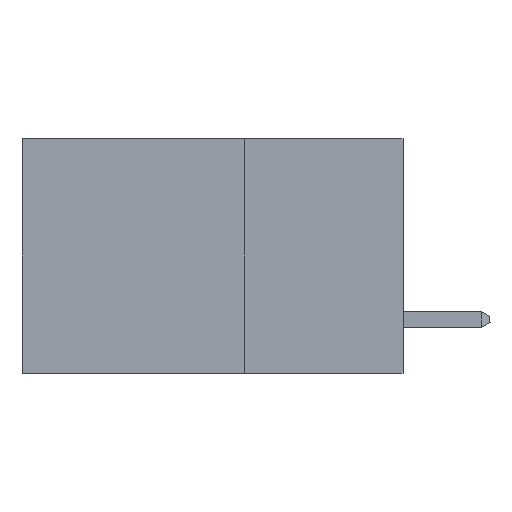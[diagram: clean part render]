
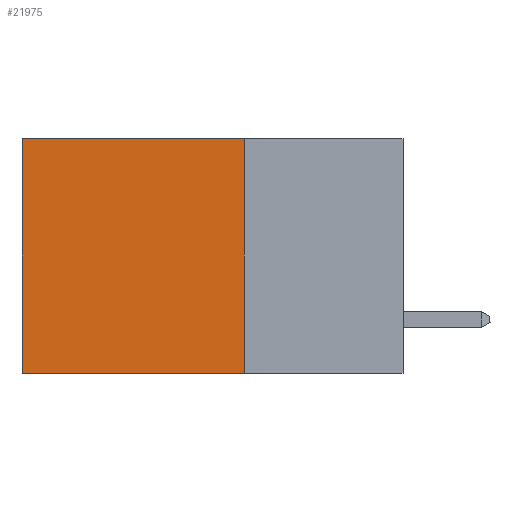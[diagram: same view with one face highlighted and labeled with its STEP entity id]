
A CAD part, left-side view. The second image highlights one B-rep face of the part: STEP entity #21975.
In plain terms, the highlighted planar face has unit normal (-1, 0, 0).
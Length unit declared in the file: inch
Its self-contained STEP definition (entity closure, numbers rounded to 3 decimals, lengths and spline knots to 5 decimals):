
#551 = EDGE_CURVE ( 'NONE', #24679, #6887, #25956, .T. ) ;
#995 = CARTESIAN_POINT ( 'NONE',  ( 0.2875, 0.25, -0.37 ) ) ;
#1259 = DIRECTION ( 'NONE',  ( 1., 0., 0. ) ) ;
#3183 = VECTOR ( 'NONE', #36712, 39.37008 ) ;
#5086 = DIRECTION ( 'NONE',  ( 0., 0., -1. ) ) ;
#6780 = VECTOR ( 'NONE', #36446, 39.37008 ) ;
#6887 = VERTEX_POINT ( 'NONE', #22088 ) ;
#7723 = DIRECTION ( 'NONE',  ( 0., 1., 0. ) ) ;
#8922 = VERTEX_POINT ( 'NONE', #23447 ) ;
#12280 = EDGE_CURVE ( 'NONE', #24679, #21773, #35137, .T. ) ;
#16312 = CARTESIAN_POINT ( 'NONE',  ( 0.2875, 0.6, 0. ) ) ;
#17929 = VECTOR ( 'NONE', #7723, 39.37008 ) ;
#19076 = EDGE_CURVE ( 'NONE', #6887, #8922, #28270, .T. ) ;
#21773 = VERTEX_POINT ( 'NONE', #31673 ) ;
#21975 = ADVANCED_FACE ( 'NONE', ( #44823 ), #28913, .F. ) ;
#22088 = CARTESIAN_POINT ( 'NONE',  ( 0.2875, 0.25, -0.37 ) ) ;
#23447 = CARTESIAN_POINT ( 'NONE',  ( 0.2875, 0.6, -0.37 ) ) ;
#23937 = LINE ( 'NONE', #16312, #3183 ) ;
#24296 = EDGE_CURVE ( 'NONE', #21773, #8922, #23937, .T. ) ;
#24679 = VERTEX_POINT ( 'NONE', #32122 ) ;
#24951 = ORIENTED_EDGE ( 'NONE', *, *, #551, .F. ) ;
#25956 = LINE ( 'NONE', #43380, #44436 ) ;
#27509 = EDGE_LOOP ( 'NONE', ( #29348, #31998, #24951, #41603 ) ) ;
#28270 = LINE ( 'NONE', #995, #17929 ) ;
#28913 = PLANE ( 'NONE',  #40176 ) ;
#29348 = ORIENTED_EDGE ( 'NONE', *, *, #24296, .T. ) ;
#30027 = DIRECTION ( 'NONE',  ( 0., 0., -1. ) ) ;
#31673 = CARTESIAN_POINT ( 'NONE',  ( 0.2875, 0.6, 0. ) ) ;
#31998 = ORIENTED_EDGE ( 'NONE', *, *, #19076, .F. ) ;
#32122 = CARTESIAN_POINT ( 'NONE',  ( 0.2875, 0.25, 0. ) ) ;
#35137 = LINE ( 'NONE', #36890, #6780 ) ;
#35907 = CARTESIAN_POINT ( 'NONE',  ( 0.2875, 0.25, 0. ) ) ;
#36446 = DIRECTION ( 'NONE',  ( 0., 1., 0. ) ) ;
#36712 = DIRECTION ( 'NONE',  ( 0., 0., -1. ) ) ;
#36890 = CARTESIAN_POINT ( 'NONE',  ( 0.2875, 0.25, 0. ) ) ;
#40176 = AXIS2_PLACEMENT_3D ( 'NONE', #35907, #1259, #5086 ) ;
#41603 = ORIENTED_EDGE ( 'NONE', *, *, #12280, .T. ) ;
#43380 = CARTESIAN_POINT ( 'NONE',  ( 0.2875, 0.25, 0. ) ) ;
#44436 = VECTOR ( 'NONE', #30027, 39.37008 ) ;
#44823 = FACE_OUTER_BOUND ( 'NONE', #27509, .T. ) ;
